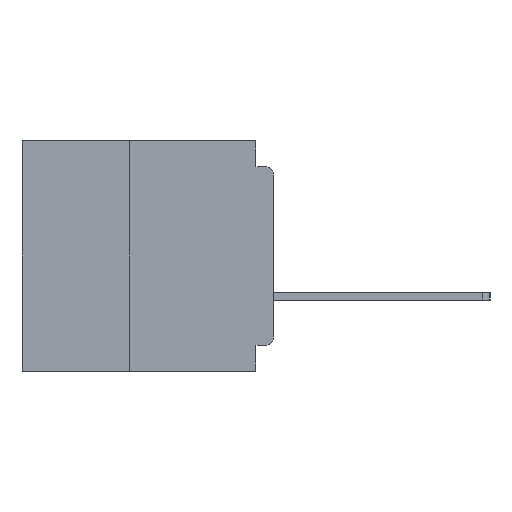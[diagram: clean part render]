
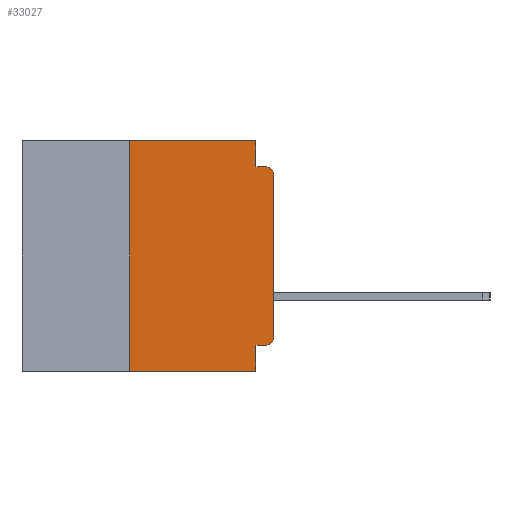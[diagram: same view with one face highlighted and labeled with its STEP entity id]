
A CAD part, left-side view. The second image highlights one B-rep face of the part: STEP entity #33027.
In plain terms, the highlighted planar face has unit normal (-1, 0, 0).
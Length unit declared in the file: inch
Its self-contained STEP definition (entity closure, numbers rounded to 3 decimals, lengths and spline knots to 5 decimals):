
#1752 = AXIS2_PLACEMENT_3D ( 'NONE', #21988, #49885, #25988 ) ;
#2464 = VERTEX_POINT ( 'NONE', #44890 ) ;
#4151 = VERTEX_POINT ( 'NONE', #16065 ) ;
#4334 = ORIENTED_EDGE ( 'NONE', *, *, #45726, .F. ) ;
#6183 = CIRCLE ( 'NONE', #1752, 0.015 ) ;
#6271 = VECTOR ( 'NONE', #45233, 39.37008 ) ;
#6960 = VERTEX_POINT ( 'NONE', #7801 ) ;
#7477 = VECTOR ( 'NONE', #23427, 39.37008 ) ;
#7510 = CARTESIAN_POINT ( 'NONE',  ( 0., 0.25, -0.4 ) ) ;
#7801 = CARTESIAN_POINT ( 'NONE',  ( 0., 0., -0.34 ) ) ;
#7994 = DIRECTION ( 'NONE',  ( -1., 0., 0. ) ) ;
#8173 = ORIENTED_EDGE ( 'NONE', *, *, #50765, .T. ) ;
#8185 = VERTEX_POINT ( 'NONE', #7510 ) ;
#8283 = CARTESIAN_POINT ( 'NONE',  ( 0., 0.031, -0.4 ) ) ;
#9081 = LINE ( 'NONE', #34154, #18423 ) ;
#9306 = ORIENTED_EDGE ( 'NONE', *, *, #28502, .F. ) ;
#10558 = ORIENTED_EDGE ( 'NONE', *, *, #41386, .F. ) ;
#11519 = EDGE_CURVE ( 'NONE', #8185, #18787, #46696, .T. ) ;
#11703 = EDGE_CURVE ( 'NONE', #29600, #6960, #6183, .T. ) ;
#11822 = VERTEX_POINT ( 'NONE', #38546 ) ;
#14798 = CARTESIAN_POINT ( 'NONE',  ( 0., 0.031, 0. ) ) ;
#15225 = CARTESIAN_POINT ( 'NONE',  ( 0., 0.015, -0.355 ) ) ;
#15996 = DIRECTION ( 'NONE',  ( 0., 0., 1. ) ) ;
#16065 = CARTESIAN_POINT ( 'NONE',  ( 0., 0.015, -0.045 ) ) ;
#16856 = LINE ( 'NONE', #21332, #6271 ) ;
#18204 = DIRECTION ( 'NONE',  ( 0., 1., 0. ) ) ;
#18423 = VECTOR ( 'NONE', #18204, 39.37008 ) ;
#18787 = VERTEX_POINT ( 'NONE', #8283 ) ;
#18954 = EDGE_CURVE ( 'NONE', #2464, #4151, #31191, .T. ) ;
#19759 = VERTEX_POINT ( 'NONE', #14798 ) ;
#19828 = CIRCLE ( 'NONE', #38193, 0.015 ) ;
#20117 = PLANE ( 'NONE',  #40124 ) ;
#20281 = ORIENTED_EDGE ( 'NONE', *, *, #18954, .F. ) ;
#21332 = CARTESIAN_POINT ( 'NONE',  ( 0., 0.031, -0.4 ) ) ;
#21988 = CARTESIAN_POINT ( 'NONE',  ( 0., 0.015, -0.34 ) ) ;
#23427 = DIRECTION ( 'NONE',  ( 0., -1., 0. ) ) ;
#24090 = DIRECTION ( 'NONE',  ( 0., 0., -1. ) ) ;
#24297 = EDGE_CURVE ( 'NONE', #8185, #27348, #49972, .T. ) ;
#24412 = CARTESIAN_POINT ( 'NONE',  ( 0., 0.031, 0. ) ) ;
#25988 = DIRECTION ( 'NONE',  ( 0., 0., -1. ) ) ;
#26084 = VECTOR ( 'NONE', #48350, 39.37008 ) ;
#26222 = EDGE_CURVE ( 'NONE', #29155, #4151, #19828, .T. ) ;
#27348 = VERTEX_POINT ( 'NONE', #46850 ) ;
#27419 = CARTESIAN_POINT ( 'NONE',  ( 0., 0.437, 0. ) ) ;
#28241 = CARTESIAN_POINT ( 'NONE',  ( 0., 0., -0.06 ) ) ;
#28502 = EDGE_CURVE ( 'NONE', #29600, #11822, #9081, .T. ) ;
#28521 = ORIENTED_EDGE ( 'NONE', *, *, #26222, .T. ) ;
#28701 = VECTOR ( 'NONE', #49314, 39.37008 ) ;
#29155 = VERTEX_POINT ( 'NONE', #28241 ) ;
#29600 = VERTEX_POINT ( 'NONE', #15225 ) ;
#31191 = LINE ( 'NONE', #41288, #51202 ) ;
#31749 = CARTESIAN_POINT ( 'NONE',  ( 0., 0.015, -0.06 ) ) ;
#33027 = ADVANCED_FACE ( 'NONE', ( #38369 ), #20117, .F. ) ;
#34154 = CARTESIAN_POINT ( 'NONE',  ( 0., 0., -0.355 ) ) ;
#35754 = DIRECTION ( 'NONE',  ( 0., 0., -1. ) ) ;
#36669 = LINE ( 'NONE', #24412, #26084 ) ;
#36850 = ORIENTED_EDGE ( 'NONE', *, *, #11519, .T. ) ;
#37249 = CARTESIAN_POINT ( 'NONE',  ( 0., 0.25, -0.4 ) ) ;
#38193 = AXIS2_PLACEMENT_3D ( 'NONE', #31749, #7994, #35754 ) ;
#38369 = FACE_OUTER_BOUND ( 'NONE', #50141, .T. ) ;
#38546 = CARTESIAN_POINT ( 'NONE',  ( 0., 0.031, -0.355 ) ) ;
#39187 = LINE ( 'NONE', #27419, #7477 ) ;
#39972 = CARTESIAN_POINT ( 'NONE',  ( 0., 0.437, 0. ) ) ;
#40124 = AXIS2_PLACEMENT_3D ( 'NONE', #39972, #48023, #24090 ) ;
#40644 = CARTESIAN_POINT ( 'NONE',  ( 0., 0.437, -0.4 ) ) ;
#41288 = CARTESIAN_POINT ( 'NONE',  ( 0., 0., -0.045 ) ) ;
#41386 = EDGE_CURVE ( 'NONE', #27348, #19759, #39187, .T. ) ;
#42173 = LINE ( 'NONE', #47864, #50294 ) ;
#42238 = ORIENTED_EDGE ( 'NONE', *, *, #45326, .F. ) ;
#44521 = ORIENTED_EDGE ( 'NONE', *, *, #24297, .F. ) ;
#44685 = DIRECTION ( 'NONE',  ( 0., -1., 0. ) ) ;
#44890 = CARTESIAN_POINT ( 'NONE',  ( 0., 0.031, -0.045 ) ) ;
#45233 = DIRECTION ( 'NONE',  ( 0., 0., -1. ) ) ;
#45326 = EDGE_CURVE ( 'NONE', #11822, #18787, #16856, .T. ) ;
#45336 = DIRECTION ( 'NONE',  ( 0., -1., 0. ) ) ;
#45448 = VECTOR ( 'NONE', #44685, 39.37008 ) ;
#45726 = EDGE_CURVE ( 'NONE', #19759, #2464, #36669, .T. ) ;
#46696 = LINE ( 'NONE', #40644, #45448 ) ;
#46850 = CARTESIAN_POINT ( 'NONE',  ( 0., 0.25, 0. ) ) ;
#47399 = ORIENTED_EDGE ( 'NONE', *, *, #11703, .T. ) ;
#47864 = CARTESIAN_POINT ( 'NONE',  ( 0., 0., 0. ) ) ;
#48023 = DIRECTION ( 'NONE',  ( 1., 0., 0. ) ) ;
#48350 = DIRECTION ( 'NONE',  ( 0., 0., -1. ) ) ;
#49314 = DIRECTION ( 'NONE',  ( 0., 0., 1. ) ) ;
#49885 = DIRECTION ( 'NONE',  ( -1., 0., 0. ) ) ;
#49972 = LINE ( 'NONE', #37249, #28701 ) ;
#50141 = EDGE_LOOP ( 'NONE', ( #8173, #28521, #20281, #4334, #10558, #44521, #36850, #42238, #9306, #47399 ) ) ;
#50294 = VECTOR ( 'NONE', #15996, 39.37008 ) ;
#50765 = EDGE_CURVE ( 'NONE', #6960, #29155, #42173, .T. ) ;
#51202 = VECTOR ( 'NONE', #45336, 39.37008 ) ;
